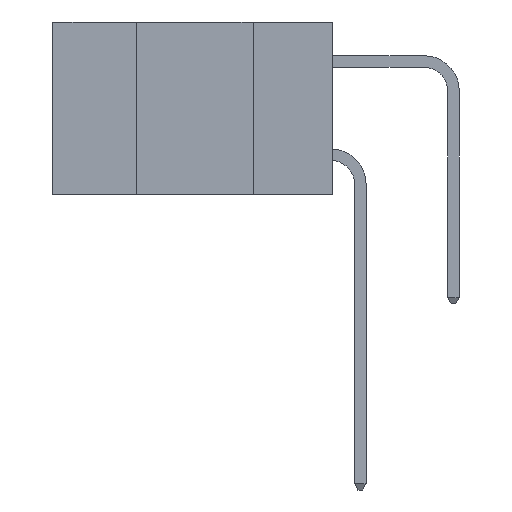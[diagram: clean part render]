
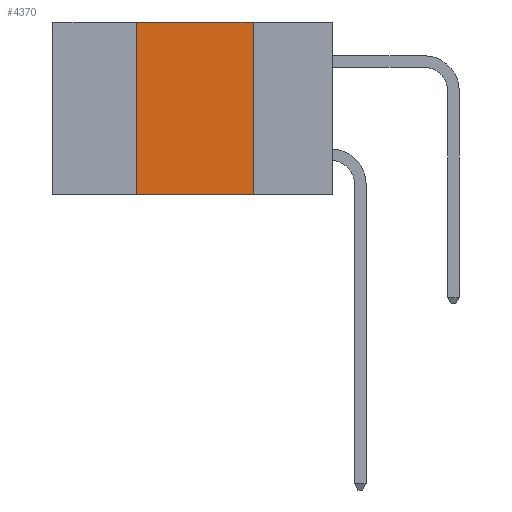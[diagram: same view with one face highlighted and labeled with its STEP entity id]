
A CAD part, left-side view. The second image highlights one B-rep face of the part: STEP entity #4370.
In plain terms, the highlighted planar face has unit normal (-1, 0, 0).
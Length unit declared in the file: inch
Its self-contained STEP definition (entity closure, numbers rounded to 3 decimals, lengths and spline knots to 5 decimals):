
#1175 = EDGE_CURVE ( 'NONE', #1683, #13131, #3558, .T. ) ;
#1625 = CARTESIAN_POINT ( 'NONE',  ( 0., 0.6, -0.37 ) ) ;
#1683 = VERTEX_POINT ( 'NONE', #5654 ) ;
#2255 = DIRECTION ( 'NONE',  ( 0., -1., 0. ) ) ;
#3422 = LINE ( 'NONE', #13280, #11890 ) ;
#3436 = VECTOR ( 'NONE', #2255, 39.37008 ) ;
#3558 = LINE ( 'NONE', #7156, #8753 ) ;
#4370 = ADVANCED_FACE ( 'NONE', ( #13689 ), #6013, .F. ) ;
#4475 = ORIENTED_EDGE ( 'NONE', *, *, #5925, .T. ) ;
#4822 = CARTESIAN_POINT ( 'NONE',  ( 0., 0.17, 0. ) ) ;
#5410 = VERTEX_POINT ( 'NONE', #4822 ) ;
#5454 = AXIS2_PLACEMENT_3D ( 'NONE', #5997, #5980, #5978 ) ;
#5654 = CARTESIAN_POINT ( 'NONE',  ( 0., 0.42, -0.37 ) ) ;
#5925 = EDGE_CURVE ( 'NONE', #1683, #10831, #6449, .T. ) ;
#5978 = DIRECTION ( 'NONE',  ( 0., 0., -1. ) ) ;
#5980 = DIRECTION ( 'NONE',  ( 1., 0., 0. ) ) ;
#5997 = CARTESIAN_POINT ( 'NONE',  ( 0., 0.6, 0. ) ) ;
#6013 = PLANE ( 'NONE',  #5454 ) ;
#6407 = EDGE_CURVE ( 'NONE', #13131, #5410, #3422, .T. ) ;
#6449 = LINE ( 'NONE', #1625, #3436 ) ;
#6742 = CARTESIAN_POINT ( 'NONE',  ( 0., 0.42, 0. ) ) ;
#7156 = CARTESIAN_POINT ( 'NONE',  ( 0., 0.42, -0.37 ) ) ;
#7429 = VECTOR ( 'NONE', #12321, 39.37008 ) ;
#7610 = ORIENTED_EDGE ( 'NONE', *, *, #1175, .F. ) ;
#7751 = LINE ( 'NONE', #12506, #7429 ) ;
#7833 = EDGE_LOOP ( 'NONE', ( #10498, #9831, #7610, #4475 ) ) ;
#8753 = VECTOR ( 'NONE', #9366, 39.37008 ) ;
#9366 = DIRECTION ( 'NONE',  ( 0., 0., 1. ) ) ;
#9831 = ORIENTED_EDGE ( 'NONE', *, *, #6407, .F. ) ;
#10498 = ORIENTED_EDGE ( 'NONE', *, *, #12613, .F. ) ;
#10831 = VERTEX_POINT ( 'NONE', #12858 ) ;
#11890 = VECTOR ( 'NONE', #13326, 39.37008 ) ;
#12321 = DIRECTION ( 'NONE',  ( 0., 0., -1. ) ) ;
#12506 = CARTESIAN_POINT ( 'NONE',  ( 0., 0.17, -0.37 ) ) ;
#12613 = EDGE_CURVE ( 'NONE', #5410, #10831, #7751, .T. ) ;
#12858 = CARTESIAN_POINT ( 'NONE',  ( 0., 0.17, -0.37 ) ) ;
#13131 = VERTEX_POINT ( 'NONE', #6742 ) ;
#13280 = CARTESIAN_POINT ( 'NONE',  ( 0., 0.6, 0. ) ) ;
#13326 = DIRECTION ( 'NONE',  ( 0., -1., 0. ) ) ;
#13689 = FACE_OUTER_BOUND ( 'NONE', #7833, .T. ) ;
